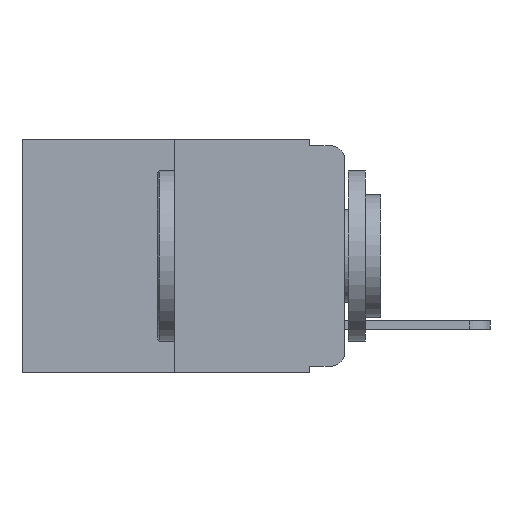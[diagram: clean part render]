
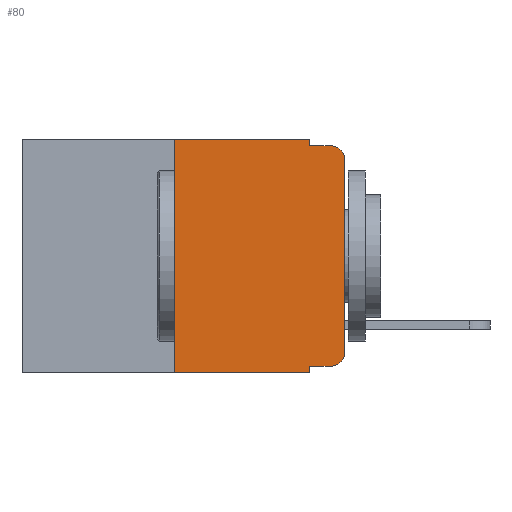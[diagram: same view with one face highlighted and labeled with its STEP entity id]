
A CAD part, left-side view. The second image highlights one B-rep face of the part: STEP entity #80.
In plain terms, the highlighted planar face has unit normal (-1, 0, 0).
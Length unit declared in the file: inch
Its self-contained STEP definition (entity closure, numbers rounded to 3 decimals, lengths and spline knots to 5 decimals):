
#52 = CARTESIAN_POINT ( 'NONE',  ( 0., 0.25, 0. ) ) ;
#59 = VERTEX_POINT ( 'NONE', #7391 ) ;
#80 = ADVANCED_FACE ( 'NONE', ( #5051 ), #566, .F. ) ;
#429 = EDGE_CURVE ( 'NONE', #11242, #4747, #5799, .T. ) ;
#514 = CARTESIAN_POINT ( 'NONE',  ( 0., 0.02, -0.313 ) ) ;
#566 = PLANE ( 'NONE',  #15775 ) ;
#1077 = DIRECTION ( 'NONE',  ( 0., 0., -1. ) ) ;
#1539 = VECTOR ( 'NONE', #12839, 39.37008 ) ;
#1759 = CARTESIAN_POINT ( 'NONE',  ( 0., 0.051, 0. ) ) ;
#1772 = DIRECTION ( 'NONE',  ( 0., -1., 0. ) ) ;
#1778 = DIRECTION ( 'NONE',  ( 1., 0., 0. ) ) ;
#1953 = CARTESIAN_POINT ( 'NONE',  ( 0., 0.051, -0.333 ) ) ;
#2089 = EDGE_CURVE ( 'NONE', #4490, #4304, #10508, .T. ) ;
#2174 = CARTESIAN_POINT ( 'NONE',  ( 0., 0.25, -0.343 ) ) ;
#2742 = LINE ( 'NONE', #6484, #9397 ) ;
#2827 = EDGE_CURVE ( 'NONE', #4304, #10245, #9535, .T. ) ;
#2878 = DIRECTION ( 'NONE',  ( 0., -1., 0. ) ) ;
#2999 = DIRECTION ( 'NONE',  ( 0., 0., -1. ) ) ;
#3195 = EDGE_CURVE ( 'NONE', #4747, #10245, #3228, .T. ) ;
#3203 = CARTESIAN_POINT ( 'NONE',  ( 0., 0., 0. ) ) ;
#3228 = LINE ( 'NONE', #9076, #1539 ) ;
#3237 = ORIENTED_EDGE ( 'NONE', *, *, #3195, .F. ) ;
#3457 = VECTOR ( 'NONE', #10431, 39.37008 ) ;
#3556 = ORIENTED_EDGE ( 'NONE', *, *, #429, .F. ) ;
#3601 = AXIS2_PLACEMENT_3D ( 'NONE', #3937, #9692, #1077 ) ;
#3937 = CARTESIAN_POINT ( 'NONE',  ( 0., 0.02, -0.03 ) ) ;
#3972 = LINE ( 'NONE', #52, #5286 ) ;
#4131 = ORIENTED_EDGE ( 'NONE', *, *, #13350, .T. ) ;
#4304 = VERTEX_POINT ( 'NONE', #5730 ) ;
#4490 = VERTEX_POINT ( 'NONE', #14517 ) ;
#4747 = VERTEX_POINT ( 'NONE', #6598 ) ;
#5051 = FACE_OUTER_BOUND ( 'NONE', #13403, .T. ) ;
#5205 = ORIENTED_EDGE ( 'NONE', *, *, #15304, .T. ) ;
#5286 = VECTOR ( 'NONE', #8548, 39.37008 ) ;
#5336 = CARTESIAN_POINT ( 'NONE',  ( 0., 0.473, -0.343 ) ) ;
#5341 = DIRECTION ( 'NONE',  ( 0., 0., -1. ) ) ;
#5551 = LINE ( 'NONE', #5336, #14763 ) ;
#5725 = ORIENTED_EDGE ( 'NONE', *, *, #2089, .T. ) ;
#5730 = CARTESIAN_POINT ( 'NONE',  ( 0., 0., -0.03 ) ) ;
#5777 = VERTEX_POINT ( 'NONE', #11302 ) ;
#5799 = LINE ( 'NONE', #1759, #8252 ) ;
#6272 = ORIENTED_EDGE ( 'NONE', *, *, #13773, .F. ) ;
#6457 = CARTESIAN_POINT ( 'NONE',  ( 0., 0.473, 0. ) ) ;
#6484 = CARTESIAN_POINT ( 'NONE',  ( 0., 0.473, 0. ) ) ;
#6598 = CARTESIAN_POINT ( 'NONE',  ( 0., 0.051, -0.01 ) ) ;
#6652 = CARTESIAN_POINT ( 'NONE',  ( 0., 0.051, -0.343 ) ) ;
#7087 = ORIENTED_EDGE ( 'NONE', *, *, #10277, .F. ) ;
#7124 = CARTESIAN_POINT ( 'NONE',  ( 0., 0.02, -0.01 ) ) ;
#7166 = VERTEX_POINT ( 'NONE', #12170 ) ;
#7391 = CARTESIAN_POINT ( 'NONE',  ( 0., 0.25, 0. ) ) ;
#7660 = DIRECTION ( 'NONE',  ( 0., 0., -1. ) ) ;
#7734 = DIRECTION ( 'NONE',  ( -1., 0., 0. ) ) ;
#8134 = CIRCLE ( 'NONE', #14050, 0.02 ) ;
#8184 = DIRECTION ( 'NONE',  ( 0., 0., 1. ) ) ;
#8252 = VECTOR ( 'NONE', #7660, 39.37008 ) ;
#8401 = VERTEX_POINT ( 'NONE', #6652 ) ;
#8548 = DIRECTION ( 'NONE',  ( 0., 0., 1. ) ) ;
#8879 = EDGE_CURVE ( 'NONE', #5777, #7166, #11476, .T. ) ;
#9076 = CARTESIAN_POINT ( 'NONE',  ( 0., 0.051, -0.01 ) ) ;
#9375 = CARTESIAN_POINT ( 'NONE',  ( 0., 0.051, 0. ) ) ;
#9397 = VECTOR ( 'NONE', #2878, 39.37008 ) ;
#9535 = CIRCLE ( 'NONE', #3601, 0.02 ) ;
#9692 = DIRECTION ( 'NONE',  ( -1., 0., 0. ) ) ;
#10245 = VERTEX_POINT ( 'NONE', #7124 ) ;
#10277 = EDGE_CURVE ( 'NONE', #12680, #59, #3972, .T. ) ;
#10431 = DIRECTION ( 'NONE',  ( 0., -1., 0. ) ) ;
#10436 = CARTESIAN_POINT ( 'NONE',  ( 0., 0.051, 0. ) ) ;
#10508 = LINE ( 'NONE', #3203, #15147 ) ;
#11242 = VERTEX_POINT ( 'NONE', #9375 ) ;
#11302 = CARTESIAN_POINT ( 'NONE',  ( 0., 0.051, -0.333 ) ) ;
#11476 = LINE ( 'NONE', #1953, #3457 ) ;
#12170 = CARTESIAN_POINT ( 'NONE',  ( 0., 0.02, -0.333 ) ) ;
#12373 = EDGE_CURVE ( 'NONE', #59, #11242, #2742, .T. ) ;
#12625 = LINE ( 'NONE', #10436, #15525 ) ;
#12680 = VERTEX_POINT ( 'NONE', #2174 ) ;
#12839 = DIRECTION ( 'NONE',  ( 0., -1., 0. ) ) ;
#12857 = DIRECTION ( 'NONE',  ( 0., 0., -1. ) ) ;
#13350 = EDGE_CURVE ( 'NONE', #12680, #8401, #5551, .T. ) ;
#13403 = EDGE_LOOP ( 'NONE', ( #5725, #14992, #3237, #3556, #13853, #7087, #4131, #6272, #14972, #5205 ) ) ;
#13773 = EDGE_CURVE ( 'NONE', #5777, #8401, #12625, .T. ) ;
#13853 = ORIENTED_EDGE ( 'NONE', *, *, #12373, .F. ) ;
#14050 = AXIS2_PLACEMENT_3D ( 'NONE', #514, #7734, #5341 ) ;
#14517 = CARTESIAN_POINT ( 'NONE',  ( 0., 0., -0.313 ) ) ;
#14763 = VECTOR ( 'NONE', #1772, 39.37008 ) ;
#14972 = ORIENTED_EDGE ( 'NONE', *, *, #8879, .T. ) ;
#14992 = ORIENTED_EDGE ( 'NONE', *, *, #2827, .T. ) ;
#15147 = VECTOR ( 'NONE', #8184, 39.37008 ) ;
#15304 = EDGE_CURVE ( 'NONE', #7166, #4490, #8134, .T. ) ;
#15525 = VECTOR ( 'NONE', #12857, 39.37008 ) ;
#15775 = AXIS2_PLACEMENT_3D ( 'NONE', #6457, #1778, #2999 ) ;
